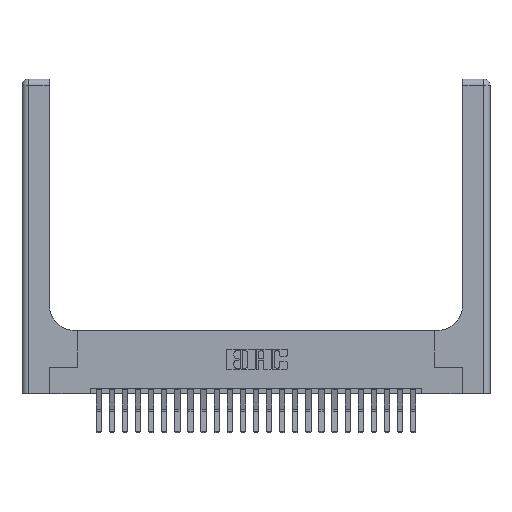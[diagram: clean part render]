
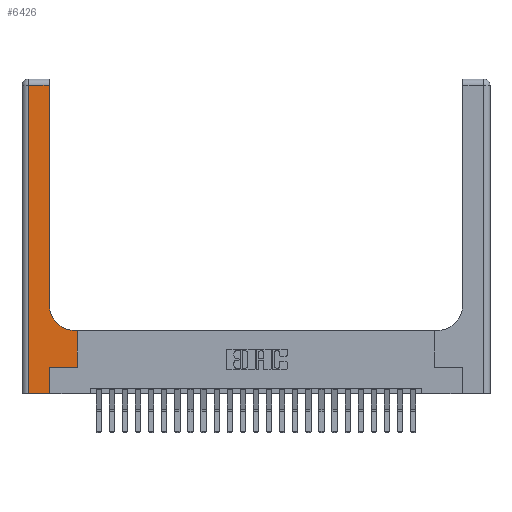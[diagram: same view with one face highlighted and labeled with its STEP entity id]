
A CAD part, top view. The second image highlights one B-rep face of the part: STEP entity #6426.
In plain terms, the highlighted planar face has unit normal (0, 0, 1).
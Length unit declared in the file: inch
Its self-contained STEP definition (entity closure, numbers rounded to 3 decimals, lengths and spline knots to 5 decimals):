
#232 = CARTESIAN_POINT ( 'NONE',  ( 0.26, 0.6, 0.37 ) ) ;
#1344 = CARTESIAN_POINT ( 'NONE',  ( 0.06, 3., 0.37 ) ) ;
#1508 = CARTESIAN_POINT ( 'NONE',  ( 0., 2.94, 0.37 ) ) ;
#1738 = EDGE_LOOP ( 'NONE', ( #22720, #11088, #2824, #16908, #2849, #3372, #19144, #20033, #12828 ) ) ;
#1947 = VECTOR ( 'NONE', #13308, 39.37008 ) ;
#2377 = VERTEX_POINT ( 'NONE', #24072 ) ;
#2716 = LINE ( 'NONE', #1344, #18845 ) ;
#2824 = ORIENTED_EDGE ( 'NONE', *, *, #3843, .T. ) ;
#2849 = ORIENTED_EDGE ( 'NONE', *, *, #3454, .T. ) ;
#2965 = CARTESIAN_POINT ( 'NONE',  ( 0.06, 2.94, 0.37 ) ) ;
#3372 = ORIENTED_EDGE ( 'NONE', *, *, #9578, .T. ) ;
#3454 = EDGE_CURVE ( 'NONE', #18004, #22157, #5541, .T. ) ;
#3729 = DIRECTION ( 'NONE',  ( 1., 0., 0. ) ) ;
#3843 = EDGE_CURVE ( 'NONE', #14163, #19010, #2716, .T. ) ;
#4053 = PLANE ( 'NONE',  #6304 ) ;
#4300 = CARTESIAN_POINT ( 'NONE',  ( 0., 3., 0.37 ) ) ;
#5087 = LINE ( 'NONE', #1508, #9930 ) ;
#5176 = CARTESIAN_POINT ( 'NONE',  ( 0.265, 0., 0.37 ) ) ;
#5541 = LINE ( 'NONE', #16655, #1947 ) ;
#5601 = VECTOR ( 'NONE', #3729, 39.37008 ) ;
#5922 = LINE ( 'NONE', #24262, #5601 ) ;
#6011 = CARTESIAN_POINT ( 'NONE',  ( 0.26, 3., 0.37 ) ) ;
#6304 = AXIS2_PLACEMENT_3D ( 'NONE', #4300, #16991, #11822 ) ;
#6426 = ADVANCED_FACE ( 'NONE', ( #15143 ), #4053, .F. ) ;
#7231 = CARTESIAN_POINT ( 'NONE',  ( 0.51, 0.85, 0.37 ) ) ;
#7818 = CARTESIAN_POINT ( 'NONE',  ( 0.265, 0.25, 0.37 ) ) ;
#8612 = CARTESIAN_POINT ( 'NONE',  ( 0.528, 0.25, 0.37 ) ) ;
#9396 = EDGE_CURVE ( 'NONE', #2377, #14163, #5087, .T. ) ;
#9484 = LINE ( 'NONE', #232, #9546 ) ;
#9546 = VECTOR ( 'NONE', #14920, 39.37008 ) ;
#9578 = EDGE_CURVE ( 'NONE', #22157, #14115, #5922, .T. ) ;
#9714 = CARTESIAN_POINT ( 'NONE',  ( 0.528, 0.6, 0.37 ) ) ;
#9718 = DIRECTION ( 'NONE',  ( 0., 1., 0. ) ) ;
#9930 = VECTOR ( 'NONE', #12610, 39.37008 ) ;
#10089 = LINE ( 'NONE', #6011, #23750 ) ;
#10372 = AXIS2_PLACEMENT_3D ( 'NONE', #7231, #20404, #13273 ) ;
#10393 = EDGE_CURVE ( 'NONE', #22192, #15741, #20969, .T. ) ;
#10563 = LINE ( 'NONE', #21756, #16269 ) ;
#11088 = ORIENTED_EDGE ( 'NONE', *, *, #9396, .T. ) ;
#11246 = EDGE_CURVE ( 'NONE', #15462, #22192, #9484, .T. ) ;
#11822 = DIRECTION ( 'NONE',  ( -1., 0., 0. ) ) ;
#11933 = EDGE_CURVE ( 'NONE', #14115, #15462, #10563, .T. ) ;
#12408 = CARTESIAN_POINT ( 'NONE',  ( 0., 0., 0.37 ) ) ;
#12610 = DIRECTION ( 'NONE',  ( -1., 0., 0. ) ) ;
#12828 = ORIENTED_EDGE ( 'NONE', *, *, #10393, .T. ) ;
#13273 = DIRECTION ( 'NONE',  ( 1., 0., 0. ) ) ;
#13308 = DIRECTION ( 'NONE',  ( 0., 1., 0. ) ) ;
#13452 = CARTESIAN_POINT ( 'NONE',  ( 0.06, 0., 0.37 ) ) ;
#13497 = CARTESIAN_POINT ( 'NONE',  ( 0.51, 0.6, 0.37 ) ) ;
#14115 = VERTEX_POINT ( 'NONE', #8612 ) ;
#14163 = VERTEX_POINT ( 'NONE', #2965 ) ;
#14920 = DIRECTION ( 'NONE',  ( -1., 0., 0. ) ) ;
#14952 = DIRECTION ( 'NONE',  ( 1., 0., 0. ) ) ;
#15143 = FACE_OUTER_BOUND ( 'NONE', #1738, .T. ) ;
#15462 = VERTEX_POINT ( 'NONE', #9714 ) ;
#15741 = VERTEX_POINT ( 'NONE', #21257 ) ;
#16269 = VECTOR ( 'NONE', #23713, 39.37008 ) ;
#16655 = CARTESIAN_POINT ( 'NONE',  ( 0.265, 0., 0.37 ) ) ;
#16908 = ORIENTED_EDGE ( 'NONE', *, *, #20641, .T. ) ;
#16991 = DIRECTION ( 'NONE',  ( 0., 0., -1. ) ) ;
#18004 = VERTEX_POINT ( 'NONE', #5176 ) ;
#18065 = LINE ( 'NONE', #12408, #20699 ) ;
#18212 = EDGE_CURVE ( 'NONE', #15741, #2377, #10089, .T. ) ;
#18845 = VECTOR ( 'NONE', #19696, 39.37008 ) ;
#19010 = VERTEX_POINT ( 'NONE', #13452 ) ;
#19144 = ORIENTED_EDGE ( 'NONE', *, *, #11933, .T. ) ;
#19696 = DIRECTION ( 'NONE',  ( 0., -1., 0. ) ) ;
#20033 = ORIENTED_EDGE ( 'NONE', *, *, #11246, .T. ) ;
#20404 = DIRECTION ( 'NONE',  ( 0., 0., -1. ) ) ;
#20641 = EDGE_CURVE ( 'NONE', #19010, #18004, #18065, .T. ) ;
#20699 = VECTOR ( 'NONE', #14952, 39.37008 ) ;
#20969 = CIRCLE ( 'NONE', #10372, 0.25 ) ;
#21257 = CARTESIAN_POINT ( 'NONE',  ( 0.26, 0.85, 0.37 ) ) ;
#21756 = CARTESIAN_POINT ( 'NONE',  ( 0.528, 0.25, 0.37 ) ) ;
#22157 = VERTEX_POINT ( 'NONE', #7818 ) ;
#22192 = VERTEX_POINT ( 'NONE', #13497 ) ;
#22720 = ORIENTED_EDGE ( 'NONE', *, *, #18212, .T. ) ;
#23713 = DIRECTION ( 'NONE',  ( 0., 1., 0. ) ) ;
#23750 = VECTOR ( 'NONE', #9718, 39.37008 ) ;
#24072 = CARTESIAN_POINT ( 'NONE',  ( 0.26, 2.94, 0.37 ) ) ;
#24262 = CARTESIAN_POINT ( 'NONE',  ( 0.265, 0.25, 0.37 ) ) ;
